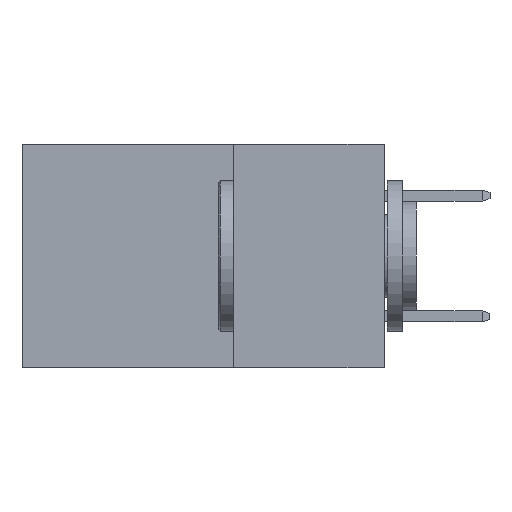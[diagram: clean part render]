
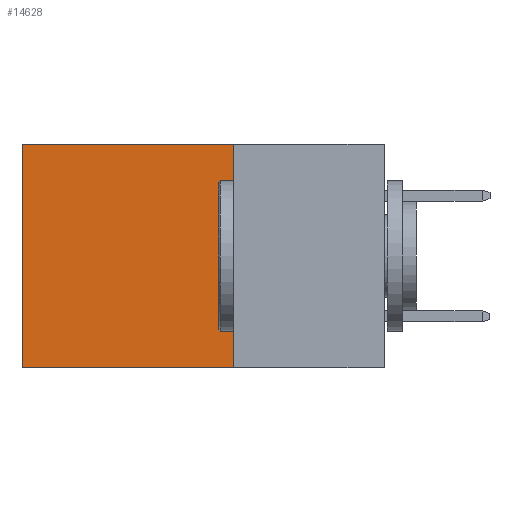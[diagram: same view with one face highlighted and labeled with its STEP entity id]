
A CAD part, left-side view. The second image highlights one B-rep face of the part: STEP entity #14628.
In plain terms, the highlighted planar face has unit normal (-1, 0, 0).
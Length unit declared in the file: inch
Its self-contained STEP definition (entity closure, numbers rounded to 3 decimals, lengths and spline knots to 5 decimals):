
#1234 = VERTEX_POINT ( 'NONE', #16405 ) ;
#1467 = DIRECTION ( 'NONE',  ( 0., 0., -1. ) ) ;
#2009 = ORIENTED_EDGE ( 'NONE', *, *, #6264, .F. ) ;
#2759 = CARTESIAN_POINT ( 'NONE',  ( 0.298, 0.25, 0. ) ) ;
#3857 = VECTOR ( 'NONE', #21408, 39.37008 ) ;
#4547 = LINE ( 'NONE', #19227, #3857 ) ;
#5612 = VERTEX_POINT ( 'NONE', #25444 ) ;
#5995 = EDGE_CURVE ( 'NONE', #24550, #5612, #24261, .T. ) ;
#6264 = EDGE_CURVE ( 'NONE', #1234, #24550, #6627, .T. ) ;
#6627 = LINE ( 'NONE', #18907, #22567 ) ;
#6985 = VECTOR ( 'NONE', #15902, 39.37008 ) ;
#7087 = DIRECTION ( 'NONE',  ( 0., 1., 0. ) ) ;
#8064 = ORIENTED_EDGE ( 'NONE', *, *, #20588, .T. ) ;
#9396 = PLANE ( 'NONE',  #13978 ) ;
#9432 = ORIENTED_EDGE ( 'NONE', *, *, #20845, .T. ) ;
#11596 = CARTESIAN_POINT ( 'NONE',  ( 0.298, 0.25, -0.37 ) ) ;
#11599 = DIRECTION ( 'NONE',  ( 0., 0., -1. ) ) ;
#12736 = VERTEX_POINT ( 'NONE', #13749 ) ;
#13749 = CARTESIAN_POINT ( 'NONE',  ( 0.298, 0.6, 0. ) ) ;
#13978 = AXIS2_PLACEMENT_3D ( 'NONE', #2759, #24504, #11599 ) ;
#14426 = VECTOR ( 'NONE', #7087, 39.37008 ) ;
#14628 = ADVANCED_FACE ( 'NONE', ( #16312 ), #9396, .F. ) ;
#15301 = EDGE_LOOP ( 'NONE', ( #8064, #26564, #2009, #9432 ) ) ;
#15902 = DIRECTION ( 'NONE',  ( 0., 1., 0. ) ) ;
#16312 = FACE_OUTER_BOUND ( 'NONE', #15301, .T. ) ;
#16405 = CARTESIAN_POINT ( 'NONE',  ( 0.298, 0.25, 0. ) ) ;
#18907 = CARTESIAN_POINT ( 'NONE',  ( 0.298, 0.25, 0. ) ) ;
#19227 = CARTESIAN_POINT ( 'NONE',  ( 0.298, 0.6, 0. ) ) ;
#20588 = EDGE_CURVE ( 'NONE', #12736, #5612, #4547, .T. ) ;
#20671 = CARTESIAN_POINT ( 'NONE',  ( 0.298, 0.25, -0.37 ) ) ;
#20835 = LINE ( 'NONE', #26550, #14426 ) ;
#20845 = EDGE_CURVE ( 'NONE', #1234, #12736, #20835, .T. ) ;
#21408 = DIRECTION ( 'NONE',  ( 0., 0., -1. ) ) ;
#22567 = VECTOR ( 'NONE', #1467, 39.37008 ) ;
#24261 = LINE ( 'NONE', #11596, #6985 ) ;
#24504 = DIRECTION ( 'NONE',  ( 1., 0., 0. ) ) ;
#24550 = VERTEX_POINT ( 'NONE', #20671 ) ;
#25444 = CARTESIAN_POINT ( 'NONE',  ( 0.298, 0.6, -0.37 ) ) ;
#26550 = CARTESIAN_POINT ( 'NONE',  ( 0.298, 0.25, 0. ) ) ;
#26564 = ORIENTED_EDGE ( 'NONE', *, *, #5995, .F. ) ;
